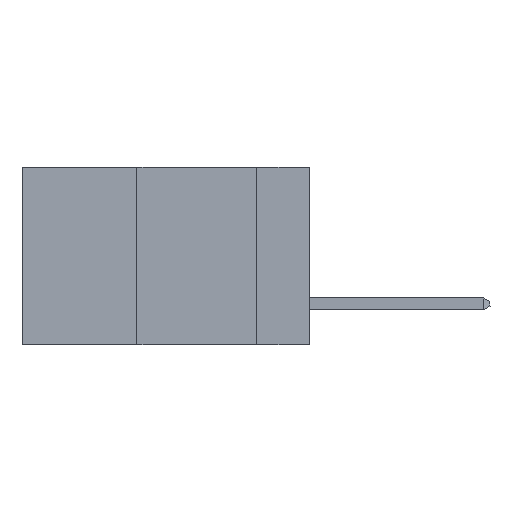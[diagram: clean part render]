
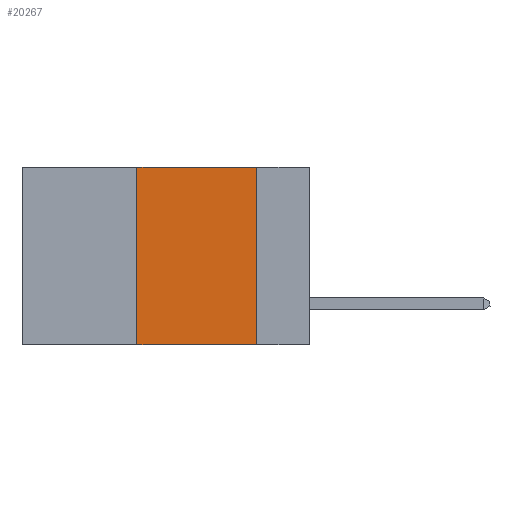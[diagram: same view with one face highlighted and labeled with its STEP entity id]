
A CAD part, left-side view. The second image highlights one B-rep face of the part: STEP entity #20267.
In plain terms, the highlighted planar face has unit normal (-1, 0, 0).
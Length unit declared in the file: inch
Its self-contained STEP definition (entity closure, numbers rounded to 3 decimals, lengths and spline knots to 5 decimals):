
#1343 = VECTOR ( 'NONE', #39469, 39.37008 ) ;
#1707 = PLANE ( 'NONE',  #24873 ) ;
#1777 = CARTESIAN_POINT ( 'NONE',  ( 0., 0.36, -0.37 ) ) ;
#2233 = ORIENTED_EDGE ( 'NONE', *, *, #23667, .F. ) ;
#5339 = DIRECTION ( 'NONE',  ( 1., 0., 0. ) ) ;
#6752 = EDGE_CURVE ( 'NONE', #9420, #40809, #8328, .T. ) ;
#7838 = ORIENTED_EDGE ( 'NONE', *, *, #7915, .F. ) ;
#7915 = EDGE_CURVE ( 'NONE', #9420, #8760, #21384, .T. ) ;
#8328 = LINE ( 'NONE', #29384, #1343 ) ;
#8760 = VERTEX_POINT ( 'NONE', #34103 ) ;
#9020 = DIRECTION ( 'NONE',  ( 0., 0., -1. ) ) ;
#9420 = VERTEX_POINT ( 'NONE', #1777 ) ;
#10042 = LINE ( 'NONE', #25187, #23620 ) ;
#10948 = CARTESIAN_POINT ( 'NONE',  ( 0., 0.6, 0. ) ) ;
#11271 = EDGE_CURVE ( 'NONE', #19546, #40809, #10042, .T. ) ;
#13325 = VECTOR ( 'NONE', #41376, 39.37008 ) ;
#18915 = CARTESIAN_POINT ( 'NONE',  ( 0., 0.36, 0. ) ) ;
#19546 = VERTEX_POINT ( 'NONE', #33610 ) ;
#20062 = ORIENTED_EDGE ( 'NONE', *, *, #11271, .F. ) ;
#20267 = ADVANCED_FACE ( 'NONE', ( #27639 ), #1707, .F. ) ;
#21384 = LINE ( 'NONE', #18915, #13325 ) ;
#23620 = VECTOR ( 'NONE', #9020, 39.37008 ) ;
#23667 = EDGE_CURVE ( 'NONE', #8760, #19546, #36863, .T. ) ;
#24153 = CARTESIAN_POINT ( 'NONE',  ( 0., 0.6, 0. ) ) ;
#24873 = AXIS2_PLACEMENT_3D ( 'NONE', #24153, #5339, #33849 ) ;
#25187 = CARTESIAN_POINT ( 'NONE',  ( 0., 0.11, 0. ) ) ;
#27639 = FACE_OUTER_BOUND ( 'NONE', #30046, .T. ) ;
#28096 = CARTESIAN_POINT ( 'NONE',  ( 0., 0.11, -0.37 ) ) ;
#29384 = CARTESIAN_POINT ( 'NONE',  ( 0., 0.6, -0.37 ) ) ;
#30046 = EDGE_LOOP ( 'NONE', ( #20062, #2233, #7838, #30663 ) ) ;
#30319 = DIRECTION ( 'NONE',  ( 0., -1., 0. ) ) ;
#30663 = ORIENTED_EDGE ( 'NONE', *, *, #6752, .T. ) ;
#31351 = VECTOR ( 'NONE', #30319, 39.37008 ) ;
#33610 = CARTESIAN_POINT ( 'NONE',  ( 0., 0.11, 0. ) ) ;
#33849 = DIRECTION ( 'NONE',  ( 0., 0., -1. ) ) ;
#34103 = CARTESIAN_POINT ( 'NONE',  ( 0., 0.36, 0. ) ) ;
#36863 = LINE ( 'NONE', #10948, #31351 ) ;
#39469 = DIRECTION ( 'NONE',  ( 0., -1., 0. ) ) ;
#40809 = VERTEX_POINT ( 'NONE', #28096 ) ;
#41376 = DIRECTION ( 'NONE',  ( 0., 0., 1. ) ) ;
